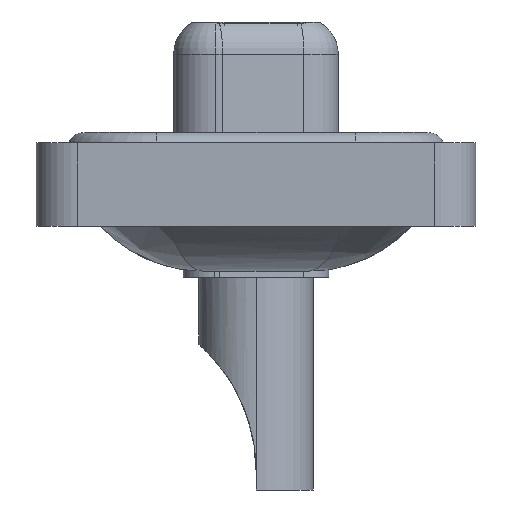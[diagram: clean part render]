
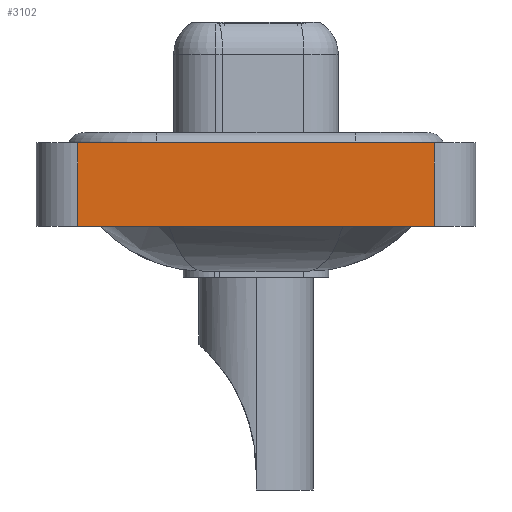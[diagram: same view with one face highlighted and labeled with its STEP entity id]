
A CAD part, left-side view. The second image highlights one B-rep face of the part: STEP entity #3102.
In plain terms, the highlighted planar face has unit normal (-1, 0, 0).
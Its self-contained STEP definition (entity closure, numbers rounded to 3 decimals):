
#752 = CARTESIAN_POINT ( 'NONE',  ( -7.25, -8.55, -3.6 ) ) ;
#1062 = CARTESIAN_POINT ( 'NONE',  ( -7.25, 8.55, -3.6 ) ) ;
#1110 = VECTOR ( 'NONE', #11365, 1000. ) ;
#1165 = CARTESIAN_POINT ( 'NONE',  ( -7.25, -8.55, 0.4 ) ) ;
#1251 = LINE ( 'NONE', #6106, #1337 ) ;
#1334 = DIRECTION ( 'NONE',  ( 0., -1., 0. ) ) ;
#1337 = VECTOR ( 'NONE', #1334, 1000. ) ;
#1811 = ORIENTED_EDGE ( 'NONE', *, *, #9860, .F. ) ;
#2913 = EDGE_CURVE ( 'NONE', #4161, #11980, #13759, .T. ) ;
#2973 = CARTESIAN_POINT ( 'NONE',  ( -7.25, 8.55, -3.6 ) ) ;
#3102 = ADVANCED_FACE ( 'NONE', ( #12865 ), #11686, .T. ) ;
#4161 = VERTEX_POINT ( 'NONE', #8523 ) ;
#4198 = EDGE_CURVE ( 'NONE', #12822, #11980, #1251, .T. ) ;
#4504 = CARTESIAN_POINT ( 'NONE',  ( -7.25, 8.55, 0.4 ) ) ;
#5111 = VECTOR ( 'NONE', #9868, 1000. ) ;
#5610 = DIRECTION ( 'NONE',  ( -1., 0., 0. ) ) ;
#5883 = LINE ( 'NONE', #15620, #7120 ) ;
#6106 = CARTESIAN_POINT ( 'NONE',  ( -7.25, -8.55, 0.4 ) ) ;
#6309 = ORIENTED_EDGE ( 'NONE', *, *, #2913, .T. ) ;
#7120 = VECTOR ( 'NONE', #14255, 1000. ) ;
#7404 = AXIS2_PLACEMENT_3D ( 'NONE', #752, #5610, #15350 ) ;
#8286 = VERTEX_POINT ( 'NONE', #1062 ) ;
#8523 = CARTESIAN_POINT ( 'NONE',  ( -7.25, -8.55, -3.6 ) ) ;
#9860 = EDGE_CURVE ( 'NONE', #8286, #12822, #12620, .T. ) ;
#9868 = DIRECTION ( 'NONE',  ( 0., 0., 1. ) ) ;
#11365 = DIRECTION ( 'NONE',  ( 0., 0., 1. ) ) ;
#11686 = PLANE ( 'NONE',  #7404 ) ;
#11980 = VERTEX_POINT ( 'NONE', #1165 ) ;
#12481 = CARTESIAN_POINT ( 'NONE',  ( -7.25, -8.55, -3.6 ) ) ;
#12620 = LINE ( 'NONE', #2973, #1110 ) ;
#12822 = VERTEX_POINT ( 'NONE', #4504 ) ;
#12865 = FACE_OUTER_BOUND ( 'NONE', #15442, .T. ) ;
#13500 = ORIENTED_EDGE ( 'NONE', *, *, #15691, .T. ) ;
#13543 = ORIENTED_EDGE ( 'NONE', *, *, #4198, .F. ) ;
#13759 = LINE ( 'NONE', #12481, #5111 ) ;
#14255 = DIRECTION ( 'NONE',  ( 0., -1., 0. ) ) ;
#15350 = DIRECTION ( 'NONE',  ( 0., 0., 1. ) ) ;
#15442 = EDGE_LOOP ( 'NONE', ( #6309, #13543, #1811, #13500 ) ) ;
#15620 = CARTESIAN_POINT ( 'NONE',  ( -7.25, -8.55, -3.6 ) ) ;
#15691 = EDGE_CURVE ( 'NONE', #8286, #4161, #5883, .T. ) ;
